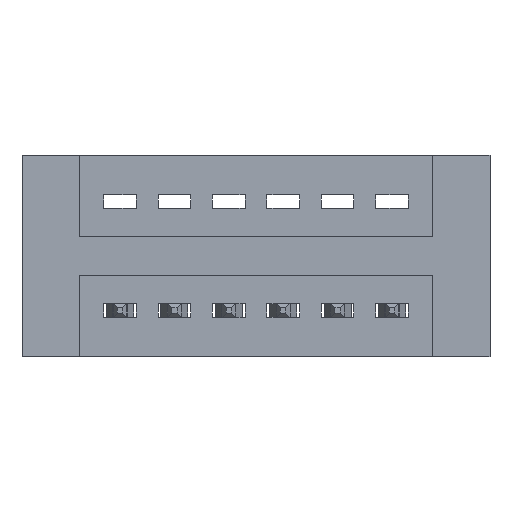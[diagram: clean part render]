
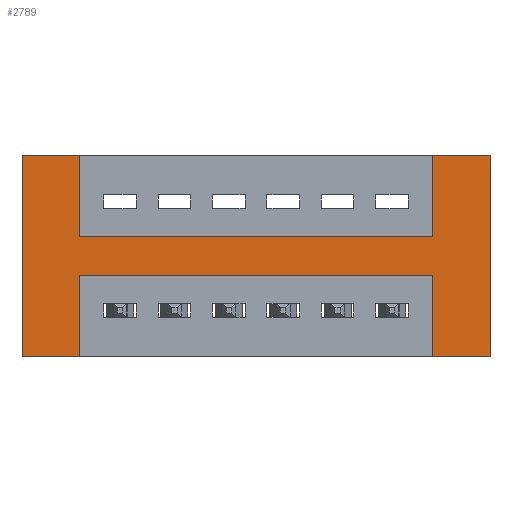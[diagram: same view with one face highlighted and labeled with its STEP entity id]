
A CAD part, front view. The second image highlights one B-rep face of the part: STEP entity #2789.
In plain terms, the highlighted planar face has unit normal (0, -1, 0).
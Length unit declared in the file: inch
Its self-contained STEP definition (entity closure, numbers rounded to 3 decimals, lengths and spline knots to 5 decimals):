
#71 = ORIENTED_EDGE ( 'NONE', *, *, #4068, .F. ) ;
#137 = VERTEX_POINT ( 'NONE', #2620 ) ;
#165 = VECTOR ( 'NONE', #4661, 39.37008 ) ;
#304 = EDGE_CURVE ( 'NONE', #137, #1209, #6760, .T. ) ;
#465 = VERTEX_POINT ( 'NONE', #791 ) ;
#525 = LINE ( 'NONE', #5745, #2552 ) ;
#568 = ORIENTED_EDGE ( 'NONE', *, *, #6019, .F. ) ;
#678 = DIRECTION ( 'NONE',  ( -1., 0., 0. ) ) ;
#791 = CARTESIAN_POINT ( 'NONE',  ( 0.3925, 0., 0. ) ) ;
#875 = CARTESIAN_POINT ( 'NONE',  ( 0., 0., 0. ) ) ;
#881 = FACE_OUTER_BOUND ( 'NONE', #8296, .T. ) ;
#965 = LINE ( 'NONE', #5580, #3402 ) ;
#1084 = ORIENTED_EDGE ( 'NONE', *, *, #7011, .F. ) ;
#1092 = ORIENTED_EDGE ( 'NONE', *, *, #1232, .F. ) ;
#1209 = VERTEX_POINT ( 'NONE', #2201 ) ;
#1232 = EDGE_CURVE ( 'NONE', #137, #465, #5334, .T. ) ;
#1337 = LINE ( 'NONE', #8247, #6872 ) ;
#1338 = CARTESIAN_POINT ( 'NONE',  ( 1.1475, 0., 0. ) ) ;
#1599 = DIRECTION ( 'NONE',  ( 0., 0., -1. ) ) ;
#1630 = CARTESIAN_POINT ( 'NONE',  ( 0.2875, 0., 0. ) ) ;
#1675 = CARTESIAN_POINT ( 'NONE',  ( 1.0425, 0., -0.15 ) ) ;
#1841 = DIRECTION ( 'NONE',  ( 0., 0., -1. ) ) ;
#1869 = DIRECTION ( 'NONE',  ( 0., -1., 0. ) ) ;
#2201 = CARTESIAN_POINT ( 'NONE',  ( 0.2875, 0., -0.37 ) ) ;
#2202 = EDGE_CURVE ( 'NONE', #7976, #3257, #7138, .T. ) ;
#2287 = ORIENTED_EDGE ( 'NONE', *, *, #4831, .F. ) ;
#2552 = VECTOR ( 'NONE', #8895, 39.37008 ) ;
#2620 = CARTESIAN_POINT ( 'NONE',  ( 0.2875, 0., 0. ) ) ;
#2760 = CARTESIAN_POINT ( 'NONE',  ( 0.3925, 0., -0.37 ) ) ;
#2775 = VECTOR ( 'NONE', #8724, 39.37008 ) ;
#2789 = ADVANCED_FACE ( 'NONE', ( #881 ), #7402, .T. ) ;
#2937 = ORIENTED_EDGE ( 'NONE', *, *, #7418, .T. ) ;
#3037 = DIRECTION ( 'NONE',  ( 1., 0., 0. ) ) ;
#3061 = CARTESIAN_POINT ( 'NONE',  ( 1.0425, 0., -0.22 ) ) ;
#3100 = DIRECTION ( 'NONE',  ( 0., 0., -1. ) ) ;
#3112 = CARTESIAN_POINT ( 'NONE',  ( 1.1475, 0., -0.37 ) ) ;
#3257 = VERTEX_POINT ( 'NONE', #6344 ) ;
#3402 = VECTOR ( 'NONE', #678, 39.37008 ) ;
#3419 = CARTESIAN_POINT ( 'NONE',  ( 1.0425, 0., -0.37 ) ) ;
#3480 = DIRECTION ( 'NONE',  ( 1., 0., 0. ) ) ;
#3546 = VECTOR ( 'NONE', #6977, 39.37008 ) ;
#3565 = VECTOR ( 'NONE', #3037, 39.37008 ) ;
#3761 = VERTEX_POINT ( 'NONE', #1675 ) ;
#3813 = LINE ( 'NONE', #8745, #5573 ) ;
#3885 = CARTESIAN_POINT ( 'NONE',  ( 1.1475, 0., 0. ) ) ;
#4015 = VECTOR ( 'NONE', #4589, 39.37008 ) ;
#4047 = ORIENTED_EDGE ( 'NONE', *, *, #2202, .F. ) ;
#4068 = EDGE_CURVE ( 'NONE', #8553, #8494, #6162, .T. ) ;
#4442 = EDGE_CURVE ( 'NONE', #3257, #1209, #8060, .T. ) ;
#4589 = DIRECTION ( 'NONE',  ( 0., 0., 1. ) ) ;
#4661 = DIRECTION ( 'NONE',  ( 0., 0., 1. ) ) ;
#4831 = EDGE_CURVE ( 'NONE', #8494, #7976, #965, .T. ) ;
#4937 = VECTOR ( 'NONE', #1599, 39.37008 ) ;
#5189 = CARTESIAN_POINT ( 'NONE',  ( 1.0425, 0., 0. ) ) ;
#5272 = ORIENTED_EDGE ( 'NONE', *, *, #8289, .F. ) ;
#5334 = LINE ( 'NONE', #875, #3565 ) ;
#5409 = ORIENTED_EDGE ( 'NONE', *, *, #4442, .F. ) ;
#5500 = EDGE_CURVE ( 'NONE', #7184, #8553, #525, .T. ) ;
#5573 = VECTOR ( 'NONE', #3100, 39.37008 ) ;
#5580 = CARTESIAN_POINT ( 'NONE',  ( 0.3925, 0., -0.22 ) ) ;
#5601 = ORIENTED_EDGE ( 'NONE', *, *, #5500, .F. ) ;
#5692 = DIRECTION ( 'NONE',  ( 1., 0., 0. ) ) ;
#5745 = CARTESIAN_POINT ( 'NONE',  ( 0., 0., -0.37 ) ) ;
#5966 = LINE ( 'NONE', #8086, #8907 ) ;
#6019 = EDGE_CURVE ( 'NONE', #465, #8425, #3813, .T. ) ;
#6162 = LINE ( 'NONE', #3419, #165 ) ;
#6214 = VERTEX_POINT ( 'NONE', #1338 ) ;
#6344 = CARTESIAN_POINT ( 'NONE',  ( 0.3925, 0., -0.37 ) ) ;
#6545 = CARTESIAN_POINT ( 'NONE',  ( 1.0425, 0., 0. ) ) ;
#6582 = CARTESIAN_POINT ( 'NONE',  ( 0.3925, 0., -0.22 ) ) ;
#6736 = EDGE_CURVE ( 'NONE', #8425, #3761, #1337, .T. ) ;
#6741 = DIRECTION ( 'NONE',  ( -1., 0., 0. ) ) ;
#6760 = LINE ( 'NONE', #1630, #4937 ) ;
#6809 = CARTESIAN_POINT ( 'NONE',  ( 0., 0., -0.37 ) ) ;
#6872 = VECTOR ( 'NONE', #5692, 39.37008 ) ;
#6977 = DIRECTION ( 'NONE',  ( 0., 0., -1. ) ) ;
#7011 = EDGE_CURVE ( 'NONE', #3761, #8540, #8112, .T. ) ;
#7080 = CARTESIAN_POINT ( 'NONE',  ( 0.3925, 0., -0.15 ) ) ;
#7137 = AXIS2_PLACEMENT_3D ( 'NONE', #7351, #1869, #1841 ) ;
#7138 = LINE ( 'NONE', #2760, #3546 ) ;
#7184 = VERTEX_POINT ( 'NONE', #3112 ) ;
#7351 = CARTESIAN_POINT ( 'NONE',  ( 0., 0., -0.37 ) ) ;
#7402 = PLANE ( 'NONE',  #7137 ) ;
#7418 = EDGE_CURVE ( 'NONE', #7184, #6214, #7538, .T. ) ;
#7538 = LINE ( 'NONE', #3885, #4015 ) ;
#7676 = ORIENTED_EDGE ( 'NONE', *, *, #6736, .F. ) ;
#7866 = VECTOR ( 'NONE', #6741, 39.37008 ) ;
#7976 = VERTEX_POINT ( 'NONE', #6582 ) ;
#8060 = LINE ( 'NONE', #6809, #7866 ) ;
#8086 = CARTESIAN_POINT ( 'NONE',  ( 0., 0., 0. ) ) ;
#8112 = LINE ( 'NONE', #5189, #2775 ) ;
#8247 = CARTESIAN_POINT ( 'NONE',  ( 0.3925, 0., -0.15 ) ) ;
#8289 = EDGE_CURVE ( 'NONE', #8540, #6214, #5966, .T. ) ;
#8296 = EDGE_LOOP ( 'NONE', ( #2937, #5272, #1084, #7676, #568, #1092, #8471, #5409, #4047, #2287, #71, #5601 ) ) ;
#8425 = VERTEX_POINT ( 'NONE', #7080 ) ;
#8471 = ORIENTED_EDGE ( 'NONE', *, *, #304, .T. ) ;
#8494 = VERTEX_POINT ( 'NONE', #3061 ) ;
#8540 = VERTEX_POINT ( 'NONE', #6545 ) ;
#8553 = VERTEX_POINT ( 'NONE', #8941 ) ;
#8724 = DIRECTION ( 'NONE',  ( 0., 0., 1. ) ) ;
#8745 = CARTESIAN_POINT ( 'NONE',  ( 0.3925, 0., 0. ) ) ;
#8895 = DIRECTION ( 'NONE',  ( -1., 0., 0. ) ) ;
#8907 = VECTOR ( 'NONE', #3480, 39.37008 ) ;
#8941 = CARTESIAN_POINT ( 'NONE',  ( 1.0425, 0., -0.37 ) ) ;
